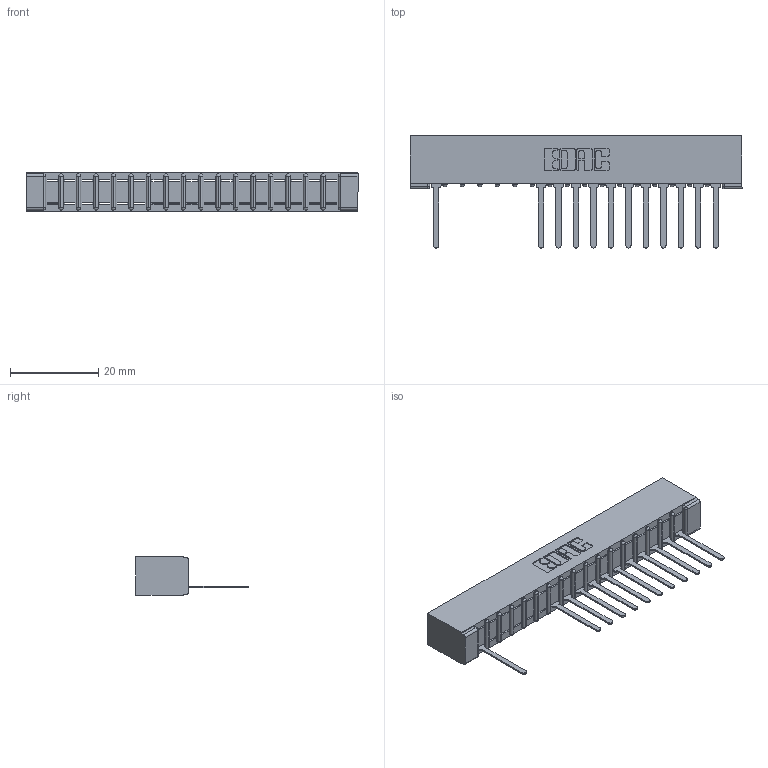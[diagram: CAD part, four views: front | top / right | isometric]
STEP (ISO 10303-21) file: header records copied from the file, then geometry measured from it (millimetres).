
FILE_DESCRIPTION (( 'STEP AP203' ), '1' );
FILE_NAME ('357-017-547-101.STEP', '2018-08-08T03:36:27', ( '' ), ( '' ), 'SwSTEP 2.0', 'SolidWorks 2016', '' );
FILE_SCHEMA (( 'CONFIG_CONTROL_DESIGN' ));
Length unit declared in the file: inch
Products named in the file (3): 307-290-001_547; 357-017-547-101; 307 Part_No Mounting Lugs
Assembly tree (13 placements, depth 2):
  357-017-547-101
    307 Part_No Mounting Lugs
    307-290-001_547  x12
Bounding box: 75.23 x 25.43 x 8.71 mm (x, y, z)
Volume: 4916.4 mm3; surface area: 7470.2 mm2
Topology: 13 solids, 13 shells, 900 faces, 2563 edges, 1642 vertices
Faces by surface type: plane 570, cylinder 294, sphere 36
Entity records: 17186 total; most frequent: CARTESIAN_POINT 2907, ORIENTED_EDGE 2898, DIRECTION 2835, EDGE_CURVE 1449, VECTOR 1103, LINE 1103, VERTEX_POINT 938, AXIS2_PLACEMENT_3D 866
